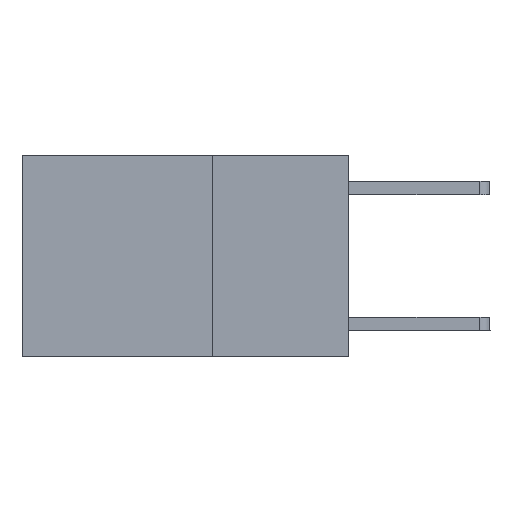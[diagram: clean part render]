
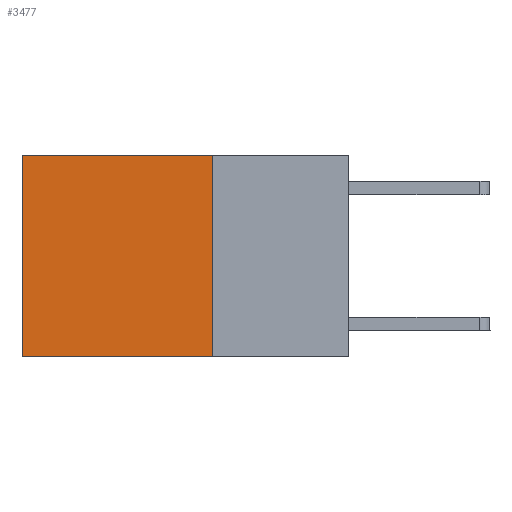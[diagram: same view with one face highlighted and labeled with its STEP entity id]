
A CAD part, left-side view. The second image highlights one B-rep face of the part: STEP entity #3477.
In plain terms, the highlighted planar face has unit normal (-1, 0, 0).
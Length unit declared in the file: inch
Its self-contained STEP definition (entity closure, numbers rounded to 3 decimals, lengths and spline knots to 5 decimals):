
#111 = DIRECTION ( 'NONE',  ( 0., 1., 0. ) ) ;
#148 = LINE ( 'NONE', #1674, #8352 ) ;
#447 = DIRECTION ( 'NONE',  ( 0., 0., -1. ) ) ;
#678 = VERTEX_POINT ( 'NONE', #6860 ) ;
#1200 = ORIENTED_EDGE ( 'NONE', *, *, #4792, .F. ) ;
#1220 = VERTEX_POINT ( 'NONE', #7015 ) ;
#1278 = VERTEX_POINT ( 'NONE', #5004 ) ;
#1499 = DIRECTION ( 'NONE',  ( 0., 0., -1. ) ) ;
#1558 = LINE ( 'NONE', #2034, #7525 ) ;
#1580 = AXIS2_PLACEMENT_3D ( 'NONE', #8264, #7810, #447 ) ;
#1674 = CARTESIAN_POINT ( 'NONE',  ( 0.2625, 0.6, 0. ) ) ;
#1758 = VERTEX_POINT ( 'NONE', #4152 ) ;
#2032 = DIRECTION ( 'NONE',  ( 0., 1., 0. ) ) ;
#2034 = CARTESIAN_POINT ( 'NONE',  ( 0.2625, 0.25, -0.37 ) ) ;
#2346 = ORIENTED_EDGE ( 'NONE', *, *, #6188, .T. ) ;
#2366 = ORIENTED_EDGE ( 'NONE', *, *, #6922, .F. ) ;
#2375 = ORIENTED_EDGE ( 'NONE', *, *, #6342, .T. ) ;
#2457 = VECTOR ( 'NONE', #111, 39.37008 ) ;
#3477 = ADVANCED_FACE ( 'NONE', ( #5411 ), #8628, .F. ) ;
#4152 = CARTESIAN_POINT ( 'NONE',  ( 0.2625, 0.6, 0. ) ) ;
#4183 = CARTESIAN_POINT ( 'NONE',  ( 0.2625, 0.25, 0. ) ) ;
#4587 = LINE ( 'NONE', #4183, #2457 ) ;
#4792 = EDGE_CURVE ( 'NONE', #1278, #1220, #1558, .T. ) ;
#5004 = CARTESIAN_POINT ( 'NONE',  ( 0.2625, 0.25, -0.37 ) ) ;
#5411 = FACE_OUTER_BOUND ( 'NONE', #8043, .T. ) ;
#6188 = EDGE_CURVE ( 'NONE', #1758, #1220, #148, .T. ) ;
#6342 = EDGE_CURVE ( 'NONE', #678, #1758, #4587, .T. ) ;
#6860 = CARTESIAN_POINT ( 'NONE',  ( 0.2625, 0.25, 0. ) ) ;
#6922 = EDGE_CURVE ( 'NONE', #678, #1278, #9875, .T. ) ;
#7015 = CARTESIAN_POINT ( 'NONE',  ( 0.2625, 0.6, -0.37 ) ) ;
#7200 = CARTESIAN_POINT ( 'NONE',  ( 0.2625, 0.25, 0. ) ) ;
#7525 = VECTOR ( 'NONE', #2032, 39.37008 ) ;
#7810 = DIRECTION ( 'NONE',  ( 1., 0., 0. ) ) ;
#8043 = EDGE_LOOP ( 'NONE', ( #2346, #1200, #2366, #2375 ) ) ;
#8264 = CARTESIAN_POINT ( 'NONE',  ( 0.2625, 0.25, 0. ) ) ;
#8352 = VECTOR ( 'NONE', #1499, 39.37008 ) ;
#8628 = PLANE ( 'NONE',  #1580 ) ;
#9405 = DIRECTION ( 'NONE',  ( 0., 0., -1. ) ) ;
#9420 = VECTOR ( 'NONE', #9405, 39.37008 ) ;
#9875 = LINE ( 'NONE', #7200, #9420 ) ;
